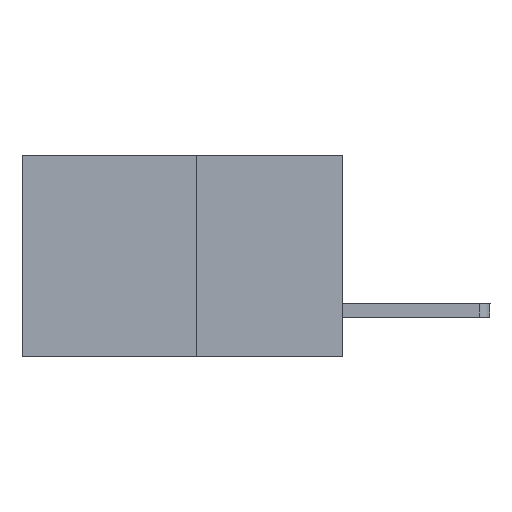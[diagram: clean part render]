
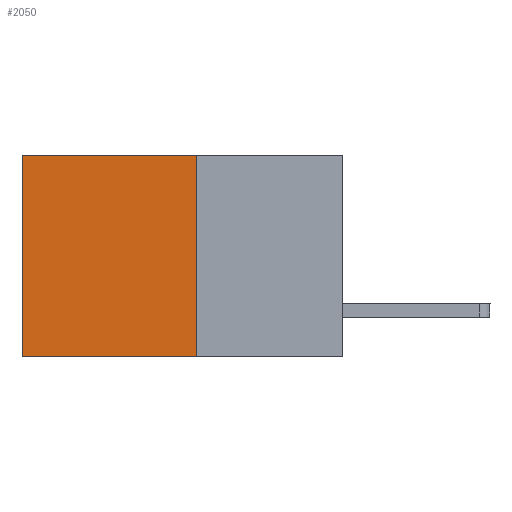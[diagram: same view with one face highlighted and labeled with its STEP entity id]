
A CAD part, left-side view. The second image highlights one B-rep face of the part: STEP entity #2050.
In plain terms, the highlighted planar face has unit normal (-1, 0, 0).
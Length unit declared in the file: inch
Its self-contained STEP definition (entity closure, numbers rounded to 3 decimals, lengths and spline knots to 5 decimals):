
#627 = VERTEX_POINT ( 'NONE', #7239 ) ;
#1182 = CARTESIAN_POINT ( 'NONE',  ( 0.277, 0.27, -0.37 ) ) ;
#1194 = DIRECTION ( 'NONE',  ( 0., 0., -1. ) ) ;
#1202 = VERTEX_POINT ( 'NONE', #8646 ) ;
#1426 = EDGE_LOOP ( 'NONE', ( #8144, #2654, #3359, #10184 ) ) ;
#1874 = LINE ( 'NONE', #10328, #2163 ) ;
#2050 = ADVANCED_FACE ( 'NONE', ( #4085 ), #9891, .F. ) ;
#2163 = VECTOR ( 'NONE', #6576, 39.37008 ) ;
#2654 = ORIENTED_EDGE ( 'NONE', *, *, #4072, .F. ) ;
#3359 = ORIENTED_EDGE ( 'NONE', *, *, #8543, .F. ) ;
#3455 = VECTOR ( 'NONE', #8427, 39.37008 ) ;
#3571 = EDGE_CURVE ( 'NONE', #9901, #627, #8735, .T. ) ;
#3944 = AXIS2_PLACEMENT_3D ( 'NONE', #5968, #5994, #4858 ) ;
#4026 = VECTOR ( 'NONE', #8746, 39.37008 ) ;
#4072 = EDGE_CURVE ( 'NONE', #5343, #1202, #1874, .T. ) ;
#4085 = FACE_OUTER_BOUND ( 'NONE', #1426, .T. ) ;
#4596 = EDGE_CURVE ( 'NONE', #627, #1202, #5810, .T. ) ;
#4858 = DIRECTION ( 'NONE',  ( 0., 0., -1. ) ) ;
#5343 = VERTEX_POINT ( 'NONE', #6374 ) ;
#5810 = LINE ( 'NONE', #9739, #3455 ) ;
#5968 = CARTESIAN_POINT ( 'NONE',  ( 0.277, 0.27, -0.37 ) ) ;
#5994 = DIRECTION ( 'NONE',  ( 1., 0., 0. ) ) ;
#6374 = CARTESIAN_POINT ( 'NONE',  ( 0.277, 0.27, -0.37 ) ) ;
#6576 = DIRECTION ( 'NONE',  ( 0., 1., 0. ) ) ;
#7239 = CARTESIAN_POINT ( 'NONE',  ( 0.277, 0.59, 0. ) ) ;
#8144 = ORIENTED_EDGE ( 'NONE', *, *, #4596, .T. ) ;
#8427 = DIRECTION ( 'NONE',  ( 0., 0., -1. ) ) ;
#8543 = EDGE_CURVE ( 'NONE', #9901, #5343, #8775, .T. ) ;
#8646 = CARTESIAN_POINT ( 'NONE',  ( 0.277, 0.59, -0.37 ) ) ;
#8735 = LINE ( 'NONE', #10853, #4026 ) ;
#8746 = DIRECTION ( 'NONE',  ( 0., 1., 0. ) ) ;
#8775 = LINE ( 'NONE', #1182, #9042 ) ;
#8941 = CARTESIAN_POINT ( 'NONE',  ( 0.277, 0.27, 0. ) ) ;
#9042 = VECTOR ( 'NONE', #1194, 39.37008 ) ;
#9739 = CARTESIAN_POINT ( 'NONE',  ( 0.277, 0.59, -0.37 ) ) ;
#9891 = PLANE ( 'NONE',  #3944 ) ;
#9901 = VERTEX_POINT ( 'NONE', #8941 ) ;
#10184 = ORIENTED_EDGE ( 'NONE', *, *, #3571, .T. ) ;
#10328 = CARTESIAN_POINT ( 'NONE',  ( 0.277, 0.27, -0.37 ) ) ;
#10853 = CARTESIAN_POINT ( 'NONE',  ( 0.277, 0.27, 0. ) ) ;
